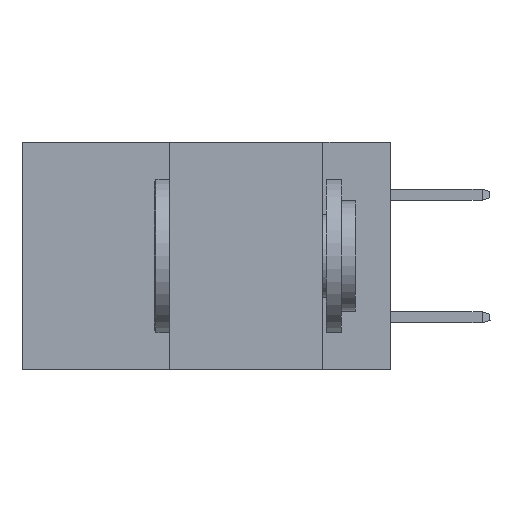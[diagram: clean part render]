
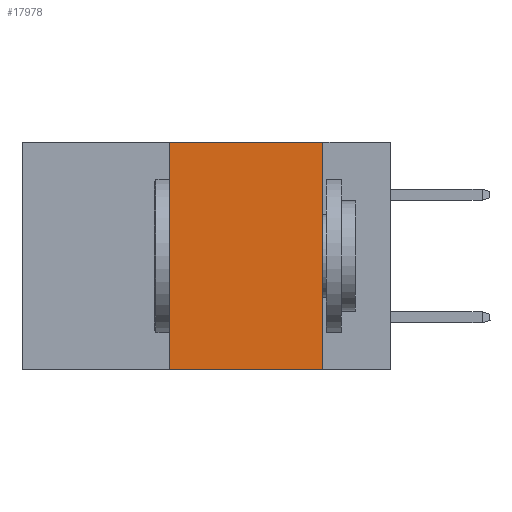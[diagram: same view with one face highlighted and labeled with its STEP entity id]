
A CAD part, left-side view. The second image highlights one B-rep face of the part: STEP entity #17978.
In plain terms, the highlighted planar face has unit normal (-1, 0, 0).
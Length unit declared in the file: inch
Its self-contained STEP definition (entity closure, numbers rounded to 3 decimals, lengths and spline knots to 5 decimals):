
#91 = CARTESIAN_POINT ( 'NONE',  ( 0., 0.6, -0.37 ) ) ;
#183 = DIRECTION ( 'NONE',  ( 0., 0., -1. ) ) ;
#280 = DIRECTION ( 'NONE',  ( 1., 0., 0. ) ) ;
#1394 = CARTESIAN_POINT ( 'NONE',  ( 0., 0.36, 0. ) ) ;
#2018 = VERTEX_POINT ( 'NONE', #17127 ) ;
#2144 = DIRECTION ( 'NONE',  ( 0., -1., 0. ) ) ;
#3141 = CARTESIAN_POINT ( 'NONE',  ( 0., 0.36, -0.37 ) ) ;
#3591 = VECTOR ( 'NONE', #16553, 39.37008 ) ;
#4650 = VERTEX_POINT ( 'NONE', #7011 ) ;
#4706 = CARTESIAN_POINT ( 'NONE',  ( 0., 0.6, 0. ) ) ;
#5923 = LINE ( 'NONE', #18452, #7982 ) ;
#6288 = DIRECTION ( 'NONE',  ( 0., -1., 0. ) ) ;
#7011 = CARTESIAN_POINT ( 'NONE',  ( 0., 0.11, -0.37 ) ) ;
#7281 = ORIENTED_EDGE ( 'NONE', *, *, #9368, .F. ) ;
#7982 = VECTOR ( 'NONE', #18265, 39.37008 ) ;
#9343 = LINE ( 'NONE', #1394, #3591 ) ;
#9368 = EDGE_CURVE ( 'NONE', #19321, #4650, #5923, .T. ) ;
#10354 = ORIENTED_EDGE ( 'NONE', *, *, #18460, .F. ) ;
#12811 = CARTESIAN_POINT ( 'NONE',  ( 0., 0.6, 0. ) ) ;
#16553 = DIRECTION ( 'NONE',  ( 0., 0., 1. ) ) ;
#16825 = LINE ( 'NONE', #91, #18170 ) ;
#17127 = CARTESIAN_POINT ( 'NONE',  ( 0., 0.36, 0. ) ) ;
#17686 = PLANE ( 'NONE',  #26470 ) ;
#17978 = ADVANCED_FACE ( 'NONE', ( #19194 ), #17686, .F. ) ;
#17981 = EDGE_CURVE ( 'NONE', #23488, #4650, #16825, .T. ) ;
#18170 = VECTOR ( 'NONE', #2144, 39.37008 ) ;
#18265 = DIRECTION ( 'NONE',  ( 0., 0., -1. ) ) ;
#18452 = CARTESIAN_POINT ( 'NONE',  ( 0., 0.11, 0. ) ) ;
#18460 = EDGE_CURVE ( 'NONE', #23488, #2018, #9343, .T. ) ;
#19194 = FACE_OUTER_BOUND ( 'NONE', #26700, .T. ) ;
#19321 = VERTEX_POINT ( 'NONE', #26148 ) ;
#19993 = ORIENTED_EDGE ( 'NONE', *, *, #27331, .F. ) ;
#21151 = VECTOR ( 'NONE', #6288, 39.37008 ) ;
#23488 = VERTEX_POINT ( 'NONE', #3141 ) ;
#23952 = ORIENTED_EDGE ( 'NONE', *, *, #17981, .T. ) ;
#26148 = CARTESIAN_POINT ( 'NONE',  ( 0., 0.11, 0. ) ) ;
#26470 = AXIS2_PLACEMENT_3D ( 'NONE', #4706, #280, #183 ) ;
#26700 = EDGE_LOOP ( 'NONE', ( #7281, #19993, #10354, #23952 ) ) ;
#26897 = LINE ( 'NONE', #12811, #21151 ) ;
#27331 = EDGE_CURVE ( 'NONE', #2018, #19321, #26897, .T. ) ;
